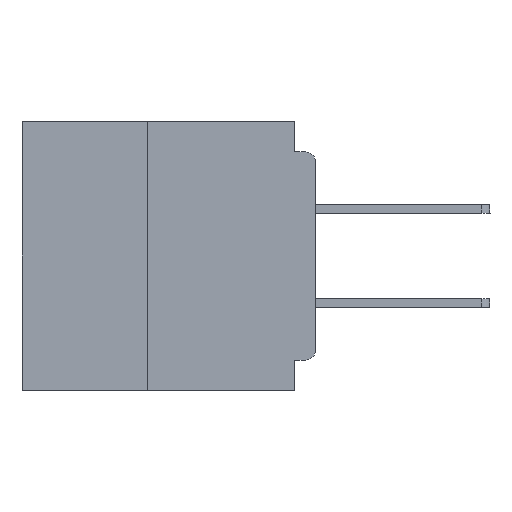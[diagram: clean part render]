
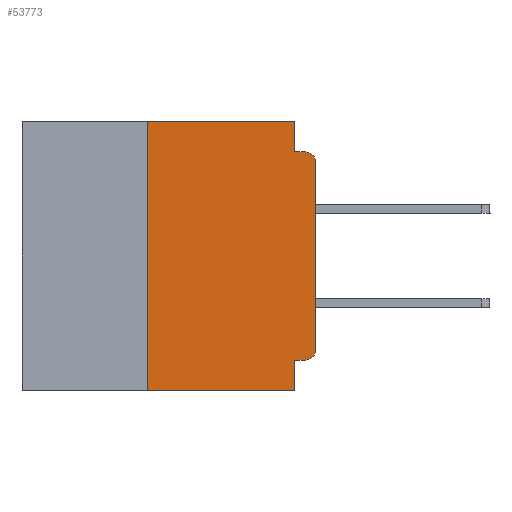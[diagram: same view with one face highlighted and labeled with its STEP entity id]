
A CAD part, left-side view. The second image highlights one B-rep face of the part: STEP entity #53773.
In plain terms, the highlighted planar face has unit normal (-1, 0, 0).
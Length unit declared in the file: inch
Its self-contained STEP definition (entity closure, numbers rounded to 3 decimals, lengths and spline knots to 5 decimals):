
#309 = CARTESIAN_POINT ( 'NONE',  ( 0., 0.031, 0. ) ) ;
#1383 = ORIENTED_EDGE ( 'NONE', *, *, #59051, .T. ) ;
#2261 = ORIENTED_EDGE ( 'NONE', *, *, #32818, .T. ) ;
#2263 = CARTESIAN_POINT ( 'NONE',  ( 0., 0.015, -0.06 ) ) ;
#4810 = EDGE_CURVE ( 'NONE', #46719, #26788, #26045, .T. ) ;
#5970 = LINE ( 'NONE', #16548, #31593 ) ;
#7385 = DIRECTION ( 'NONE',  ( 0., 0., -1. ) ) ;
#8049 = EDGE_CURVE ( 'NONE', #26788, #43294, #64296, .T. ) ;
#8105 = DIRECTION ( 'NONE',  ( 0., -1., 0. ) ) ;
#8678 = AXIS2_PLACEMENT_3D ( 'NONE', #48168, #17802, #53259 ) ;
#8844 = ORIENTED_EDGE ( 'NONE', *, *, #15032, .F. ) ;
#9744 = VERTEX_POINT ( 'NONE', #63073 ) ;
#11874 = VERTEX_POINT ( 'NONE', #12175 ) ;
#12175 = CARTESIAN_POINT ( 'NONE',  ( 0., 0.25, -0.4 ) ) ;
#12687 = PLANE ( 'NONE',  #8678 ) ;
#15032 = EDGE_CURVE ( 'NONE', #11874, #46719, #19357, .T. ) ;
#15132 = VERTEX_POINT ( 'NONE', #34720 ) ;
#16548 = CARTESIAN_POINT ( 'NONE',  ( 0., 0.031, -0.4 ) ) ;
#17802 = DIRECTION ( 'NONE',  ( 1., 0., 0. ) ) ;
#18674 = VERTEX_POINT ( 'NONE', #36666 ) ;
#19201 = EDGE_CURVE ( 'NONE', #52056, #18674, #53386, .T. ) ;
#19357 = LINE ( 'NONE', #59463, #44731 ) ;
#20568 = ORIENTED_EDGE ( 'NONE', *, *, #19201, .F. ) ;
#21064 = VERTEX_POINT ( 'NONE', #53344 ) ;
#21657 = CIRCLE ( 'NONE', #57755, 0.015 ) ;
#21691 = DIRECTION ( 'NONE',  ( 0., 0., -1. ) ) ;
#21842 = VERTEX_POINT ( 'NONE', #29838 ) ;
#22781 = CARTESIAN_POINT ( 'NONE',  ( 0., 0.015, -0.34 ) ) ;
#23917 = VECTOR ( 'NONE', #39496, 39.37008 ) ;
#24469 = DIRECTION ( 'NONE',  ( 0., -1., 0. ) ) ;
#24667 = CARTESIAN_POINT ( 'NONE',  ( 0., 0.25, 0. ) ) ;
#25142 = CARTESIAN_POINT ( 'NONE',  ( 0., 0.437, 0. ) ) ;
#26045 = LINE ( 'NONE', #25142, #63240 ) ;
#26788 = VERTEX_POINT ( 'NONE', #309 ) ;
#27909 = DIRECTION ( 'NONE',  ( 0., 0., -1. ) ) ;
#28646 = EDGE_CURVE ( 'NONE', #11874, #15132, #62240, .T. ) ;
#29838 = CARTESIAN_POINT ( 'NONE',  ( 0., 0.015, -0.045 ) ) ;
#30700 = EDGE_CURVE ( 'NONE', #43294, #21842, #50935, .T. ) ;
#31272 = VECTOR ( 'NONE', #49257, 39.37008 ) ;
#31563 = EDGE_LOOP ( 'NONE', ( #1383, #2261, #48040, #45172, #45661, #8844, #41903, #52763, #20568, #37203 ) ) ;
#31593 = VECTOR ( 'NONE', #21691, 39.37008 ) ;
#32818 = EDGE_CURVE ( 'NONE', #21064, #21842, #21657, .T. ) ;
#33329 = FACE_OUTER_BOUND ( 'NONE', #31563, .T. ) ;
#34427 = CARTESIAN_POINT ( 'NONE',  ( 0., 0.031, 0. ) ) ;
#34720 = CARTESIAN_POINT ( 'NONE',  ( 0., 0.031, -0.4 ) ) ;
#35411 = VECTOR ( 'NONE', #8105, 39.37008 ) ;
#35474 = EDGE_CURVE ( 'NONE', #18674, #15132, #5970, .T. ) ;
#36666 = CARTESIAN_POINT ( 'NONE',  ( 0., 0.031, -0.355 ) ) ;
#37203 = ORIENTED_EDGE ( 'NONE', *, *, #53163, .T. ) ;
#38018 = DIRECTION ( 'NONE',  ( -1., 0., 0. ) ) ;
#39496 = DIRECTION ( 'NONE',  ( 0., 0., -1. ) ) ;
#39853 = AXIS2_PLACEMENT_3D ( 'NONE', #22781, #58186, #27909 ) ;
#41903 = ORIENTED_EDGE ( 'NONE', *, *, #28646, .T. ) ;
#43294 = VERTEX_POINT ( 'NONE', #65674 ) ;
#44731 = VECTOR ( 'NONE', #64541, 39.37008 ) ;
#45172 = ORIENTED_EDGE ( 'NONE', *, *, #8049, .F. ) ;
#45661 = ORIENTED_EDGE ( 'NONE', *, *, #4810, .F. ) ;
#46719 = VERTEX_POINT ( 'NONE', #24667 ) ;
#47745 = VECTOR ( 'NONE', #54317, 39.37008 ) ;
#48040 = ORIENTED_EDGE ( 'NONE', *, *, #30700, .F. ) ;
#48168 = CARTESIAN_POINT ( 'NONE',  ( 0., 0.437, 0. ) ) ;
#48802 = CARTESIAN_POINT ( 'NONE',  ( 0., 0.437, -0.4 ) ) ;
#49257 = DIRECTION ( 'NONE',  ( 0., 1., 0. ) ) ;
#49446 = CARTESIAN_POINT ( 'NONE',  ( 0., 0., 0. ) ) ;
#50935 = LINE ( 'NONE', #59178, #47745 ) ;
#52056 = VERTEX_POINT ( 'NONE', #62972 ) ;
#52763 = ORIENTED_EDGE ( 'NONE', *, *, #35474, .F. ) ;
#53163 = EDGE_CURVE ( 'NONE', #52056, #9744, #59513, .T. ) ;
#53259 = DIRECTION ( 'NONE',  ( 0., 0., -1. ) ) ;
#53344 = CARTESIAN_POINT ( 'NONE',  ( 0., 0., -0.06 ) ) ;
#53386 = LINE ( 'NONE', #60864, #31272 ) ;
#53773 = ADVANCED_FACE ( 'NONE', ( #33329 ), #12687, .F. ) ;
#54317 = DIRECTION ( 'NONE',  ( 0., -1., 0. ) ) ;
#54525 = DIRECTION ( 'NONE',  ( 0., 0., 1. ) ) ;
#57755 = AXIS2_PLACEMENT_3D ( 'NONE', #2263, #38018, #7385 ) ;
#58186 = DIRECTION ( 'NONE',  ( -1., 0., 0. ) ) ;
#59051 = EDGE_CURVE ( 'NONE', #9744, #21064, #64163, .T. ) ;
#59178 = CARTESIAN_POINT ( 'NONE',  ( 0., 0., -0.045 ) ) ;
#59463 = CARTESIAN_POINT ( 'NONE',  ( 0., 0.25, -0.4 ) ) ;
#59513 = CIRCLE ( 'NONE', #39853, 0.015 ) ;
#60864 = CARTESIAN_POINT ( 'NONE',  ( 0., 0., -0.355 ) ) ;
#62240 = LINE ( 'NONE', #48802, #35411 ) ;
#62587 = VECTOR ( 'NONE', #54525, 39.37008 ) ;
#62972 = CARTESIAN_POINT ( 'NONE',  ( 0., 0.015, -0.355 ) ) ;
#63073 = CARTESIAN_POINT ( 'NONE',  ( 0., 0., -0.34 ) ) ;
#63240 = VECTOR ( 'NONE', #24469, 39.37008 ) ;
#64163 = LINE ( 'NONE', #49446, #62587 ) ;
#64296 = LINE ( 'NONE', #34427, #23917 ) ;
#64541 = DIRECTION ( 'NONE',  ( 0., 0., 1. ) ) ;
#65674 = CARTESIAN_POINT ( 'NONE',  ( 0., 0.031, -0.045 ) ) ;
